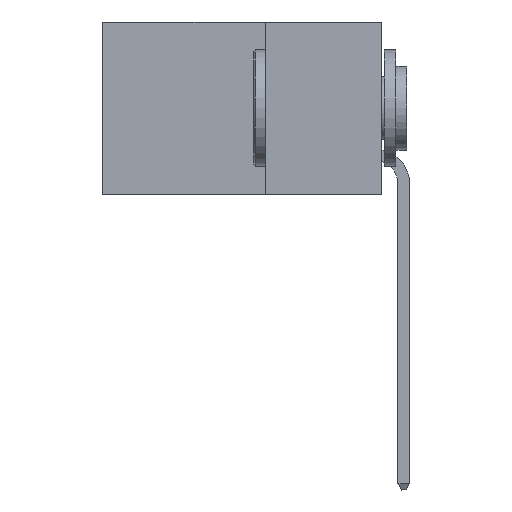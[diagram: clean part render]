
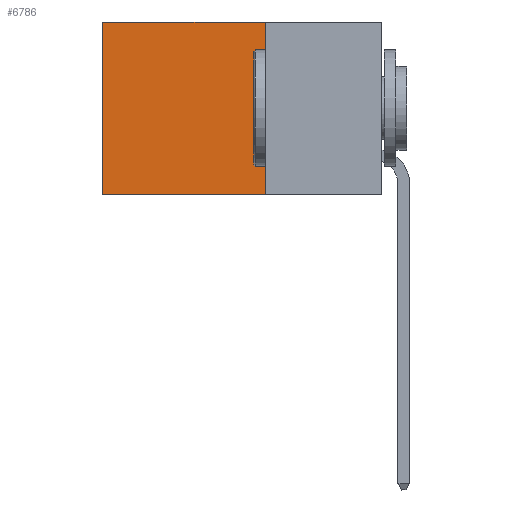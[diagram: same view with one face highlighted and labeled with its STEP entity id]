
A CAD part, left-side view. The second image highlights one B-rep face of the part: STEP entity #6786.
In plain terms, the highlighted planar face has unit normal (-1, 0, 0).
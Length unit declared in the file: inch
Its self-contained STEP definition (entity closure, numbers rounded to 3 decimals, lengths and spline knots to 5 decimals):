
#460 = VECTOR ( 'NONE', #6673, 39.37008 ) ;
#857 = LINE ( 'NONE', #12563, #21577 ) ;
#2639 = DIRECTION ( 'NONE',  ( 0., 1., 0. ) ) ;
#3767 = VERTEX_POINT ( 'NONE', #12452 ) ;
#3805 = VECTOR ( 'NONE', #2639, 39.37008 ) ;
#4673 = CARTESIAN_POINT ( 'NONE',  ( 0.2875, 0.6, 0. ) ) ;
#5194 = LINE ( 'NONE', #12930, #25866 ) ;
#6170 = EDGE_CURVE ( 'NONE', #8691, #22286, #20612, .T. ) ;
#6673 = DIRECTION ( 'NONE',  ( 0., 0., -1. ) ) ;
#6786 = ADVANCED_FACE ( 'NONE', ( #15070 ), #25550, .F. ) ;
#6969 = CARTESIAN_POINT ( 'NONE',  ( 0.2875, 0.25, 0. ) ) ;
#7516 = ORIENTED_EDGE ( 'NONE', *, *, #6170, .F. ) ;
#7989 = LINE ( 'NONE', #4673, #460 ) ;
#8691 = VERTEX_POINT ( 'NONE', #10741 ) ;
#8922 = VERTEX_POINT ( 'NONE', #13206 ) ;
#10741 = CARTESIAN_POINT ( 'NONE',  ( 0.2875, 0.25, -0.37 ) ) ;
#10816 = ORIENTED_EDGE ( 'NONE', *, *, #23612, .F. ) ;
#11519 = EDGE_CURVE ( 'NONE', #3767, #22286, #7989, .T. ) ;
#12452 = CARTESIAN_POINT ( 'NONE',  ( 0.2875, 0.6, 0. ) ) ;
#12563 = CARTESIAN_POINT ( 'NONE',  ( 0.2875, 0.25, 0. ) ) ;
#12599 = EDGE_LOOP ( 'NONE', ( #25138, #7516, #10816, #23786 ) ) ;
#12930 = CARTESIAN_POINT ( 'NONE',  ( 0.2875, 0.25, 0. ) ) ;
#13179 = DIRECTION ( 'NONE',  ( 1., 0., 0. ) ) ;
#13206 = CARTESIAN_POINT ( 'NONE',  ( 0.2875, 0.25, 0. ) ) ;
#15070 = FACE_OUTER_BOUND ( 'NONE', #12599, .T. ) ;
#15372 = DIRECTION ( 'NONE',  ( 0., 0., -1. ) ) ;
#19424 = DIRECTION ( 'NONE',  ( 0., 0., -1. ) ) ;
#19811 = DIRECTION ( 'NONE',  ( 0., 1., 0. ) ) ;
#20612 = LINE ( 'NONE', #25283, #3805 ) ;
#21577 = VECTOR ( 'NONE', #19811, 39.37008 ) ;
#22132 = AXIS2_PLACEMENT_3D ( 'NONE', #6969, #13179, #15372 ) ;
#22286 = VERTEX_POINT ( 'NONE', #23899 ) ;
#23612 = EDGE_CURVE ( 'NONE', #8922, #8691, #5194, .T. ) ;
#23786 = ORIENTED_EDGE ( 'NONE', *, *, #25493, .T. ) ;
#23899 = CARTESIAN_POINT ( 'NONE',  ( 0.2875, 0.6, -0.37 ) ) ;
#25138 = ORIENTED_EDGE ( 'NONE', *, *, #11519, .T. ) ;
#25283 = CARTESIAN_POINT ( 'NONE',  ( 0.2875, 0.25, -0.37 ) ) ;
#25493 = EDGE_CURVE ( 'NONE', #8922, #3767, #857, .T. ) ;
#25550 = PLANE ( 'NONE',  #22132 ) ;
#25866 = VECTOR ( 'NONE', #19424, 39.37008 ) ;
